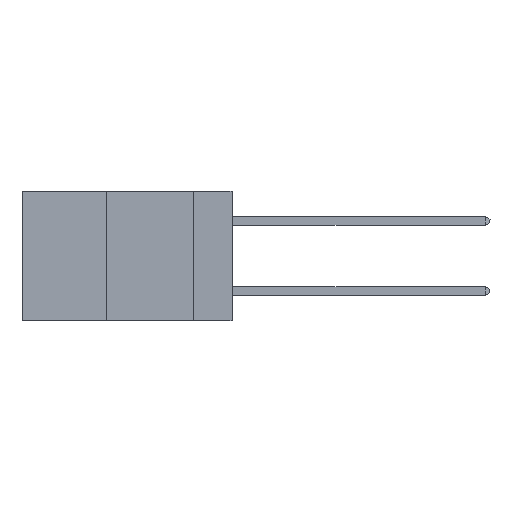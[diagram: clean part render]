
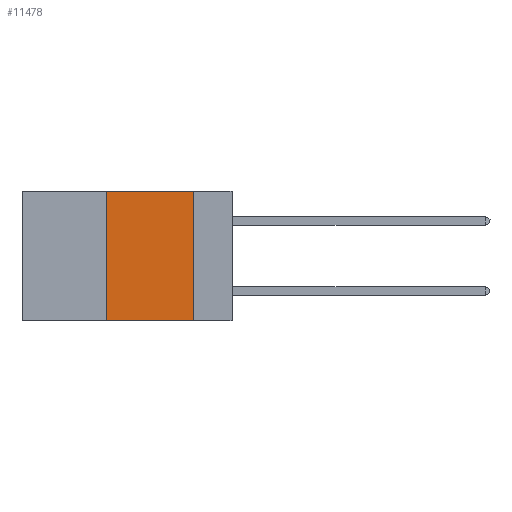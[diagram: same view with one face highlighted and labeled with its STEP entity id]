
A CAD part, left-side view. The second image highlights one B-rep face of the part: STEP entity #11478.
In plain terms, the highlighted planar face has unit normal (-1, 0, 0).
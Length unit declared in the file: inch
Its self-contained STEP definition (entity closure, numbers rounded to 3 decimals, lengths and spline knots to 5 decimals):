
#316 = FACE_OUTER_BOUND ( 'NONE', #17356, .T. ) ;
#354 = CARTESIAN_POINT ( 'NONE',  ( 0., 0.11, -0.37 ) ) ;
#410 = VERTEX_POINT ( 'NONE', #354 ) ;
#957 = DIRECTION ( 'NONE',  ( 0., -1., 0. ) ) ;
#1010 = EDGE_CURVE ( 'NONE', #26410, #410, #10489, .T. ) ;
#1527 = VERTEX_POINT ( 'NONE', #14994 ) ;
#1536 = CARTESIAN_POINT ( 'NONE',  ( 0., 0.36, 0. ) ) ;
#2974 = CARTESIAN_POINT ( 'NONE',  ( 0., 0.11, 0. ) ) ;
#3634 = CARTESIAN_POINT ( 'NONE',  ( 0., 0.6, 0. ) ) ;
#4452 = EDGE_CURVE ( 'NONE', #1527, #410, #4718, .T. ) ;
#4718 = LINE ( 'NONE', #2974, #12842 ) ;
#5350 = EDGE_CURVE ( 'NONE', #26410, #17882, #22294, .T. ) ;
#5688 = VECTOR ( 'NONE', #957, 39.37008 ) ;
#8671 = DIRECTION ( 'NONE',  ( 0., 0., 1. ) ) ;
#8926 = ORIENTED_EDGE ( 'NONE', *, *, #1010, .T. ) ;
#10254 = DIRECTION ( 'NONE',  ( 0., 0., -1. ) ) ;
#10363 = CARTESIAN_POINT ( 'NONE',  ( 0., 0.36, -0.37 ) ) ;
#10489 = LINE ( 'NONE', #20687, #27771 ) ;
#11466 = CARTESIAN_POINT ( 'NONE',  ( 0., 0.6, 0. ) ) ;
#11478 = ADVANCED_FACE ( 'NONE', ( #316 ), #24393, .F. ) ;
#12215 = EDGE_CURVE ( 'NONE', #17882, #1527, #26997, .T. ) ;
#12842 = VECTOR ( 'NONE', #10254, 39.37008 ) ;
#12997 = DIRECTION ( 'NONE',  ( 0., 0., -1. ) ) ;
#14994 = CARTESIAN_POINT ( 'NONE',  ( 0., 0.11, 0. ) ) ;
#16267 = ORIENTED_EDGE ( 'NONE', *, *, #12215, .F. ) ;
#17356 = EDGE_LOOP ( 'NONE', ( #25804, #16267, #29089, #8926 ) ) ;
#17882 = VERTEX_POINT ( 'NONE', #27486 ) ;
#18408 = AXIS2_PLACEMENT_3D ( 'NONE', #3634, #26691, #12997 ) ;
#19016 = VECTOR ( 'NONE', #8671, 39.37008 ) ;
#20687 = CARTESIAN_POINT ( 'NONE',  ( 0., 0.6, -0.37 ) ) ;
#20989 = DIRECTION ( 'NONE',  ( 0., -1., 0. ) ) ;
#22294 = LINE ( 'NONE', #1536, #19016 ) ;
#24393 = PLANE ( 'NONE',  #18408 ) ;
#25804 = ORIENTED_EDGE ( 'NONE', *, *, #4452, .F. ) ;
#26410 = VERTEX_POINT ( 'NONE', #10363 ) ;
#26691 = DIRECTION ( 'NONE',  ( 1., 0., 0. ) ) ;
#26997 = LINE ( 'NONE', #11466, #5688 ) ;
#27486 = CARTESIAN_POINT ( 'NONE',  ( 0., 0.36, 0. ) ) ;
#27771 = VECTOR ( 'NONE', #20989, 39.37008 ) ;
#29089 = ORIENTED_EDGE ( 'NONE', *, *, #5350, .F. ) ;
